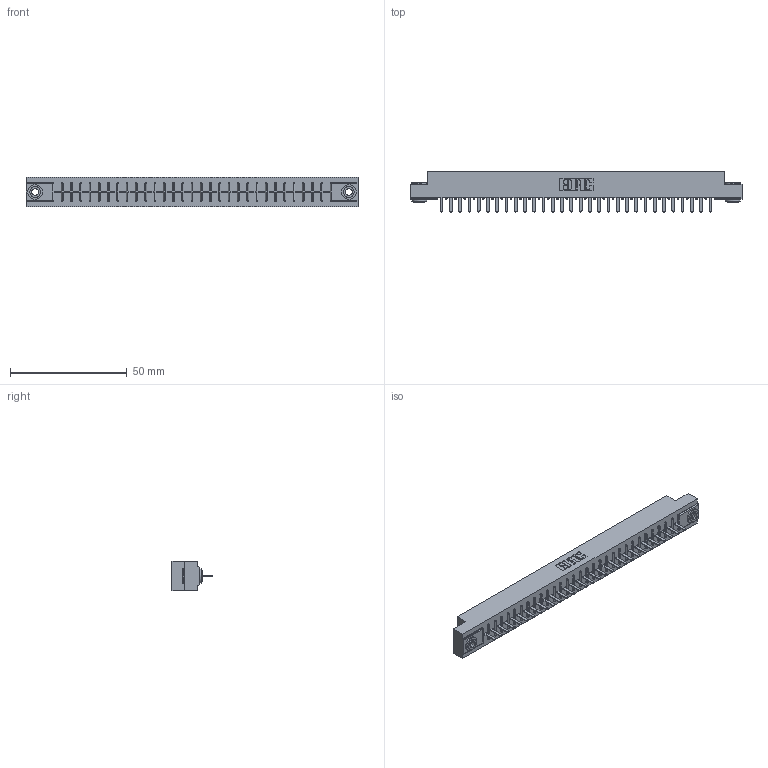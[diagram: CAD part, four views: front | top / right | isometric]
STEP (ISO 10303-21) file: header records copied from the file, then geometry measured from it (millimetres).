
FILE_DESCRIPTION (( 'STEP AP203' ), '1' );
FILE_NAME ('306-030-420-103.STEP', '2020-09-22T01:10:48', ( '' ), ( '' ), 'SwSTEP 2.0', 'SolidWorks 2020', '' );
FILE_SCHEMA (( 'CONFIG_CONTROL_DESIGN' ));
Length unit declared in the file: inch
Products named in the file (4): 306-030-420-103; 306-290-001_120; 306 Part_.156 Dia; 345-250-002_345-250-002-102
Assembly tree (33 placements, depth 2):
  306-030-420-103
    306 Part_.156 Dia
    306-290-001_120  x30
    345-250-002_345-250-002-102  x2
Bounding box: 141.88 x 17.12 x 12.7 mm (x, y, z)
Volume: 15584.1 mm3; surface area: 16137.6 mm2
Topology: 33 solids, 33 shells, 2268 faces, 6338 edges, 4060 vertices
Faces by surface type: plane 1502, cylinder 638, sphere 120, cone 8
Entity records: 30552 total; most frequent: CARTESIAN_POINT 5106, ORIENTED_EDGE 5052, DIRECTION 5050, EDGE_CURVE 2526, VECTOR 1962, LINE 1962, VERTEX_POINT 1600, AXIS2_PLACEMENT_3D 1544
